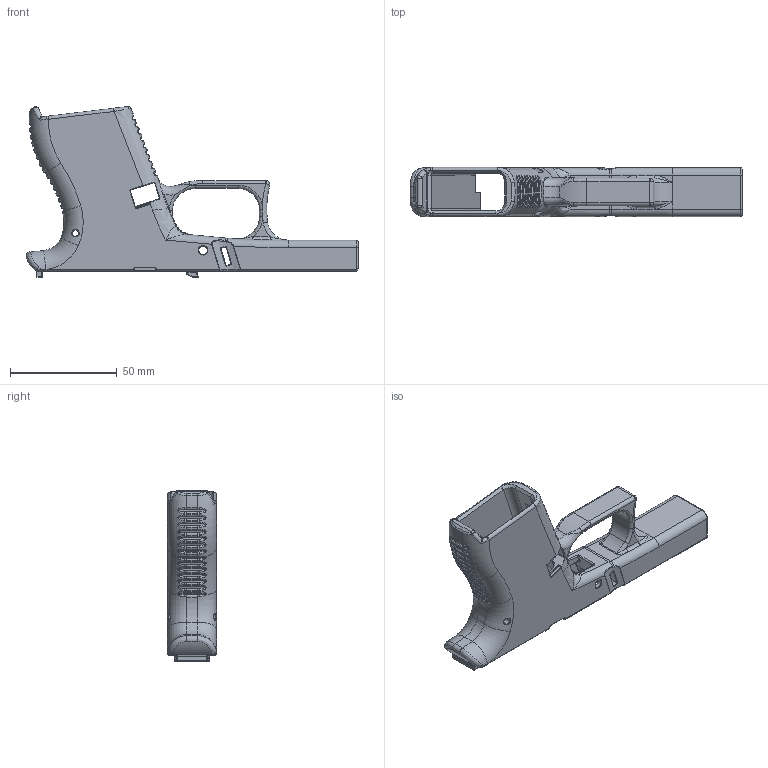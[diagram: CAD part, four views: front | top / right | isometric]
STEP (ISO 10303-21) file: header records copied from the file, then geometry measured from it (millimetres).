
FILE_DESCRIPTION(/* description */ (''),/* implementation_level */ '2;1');
FILE_NAME(/* name */ '23eda23c-9b73-40d3-b3ed-fe795d71b097.stp',/* time_stamp */ '2019-05-26T20:03:47-04:00',/* author */ ('suzuki450ltr'),/* organization */ (''),/* preprocessor_version */ 'ST-DEVELOPER v18',/* originating_system */ 'Autodesk Translation Framework v8.2.0.1029',/* authorisation */ '');
FILE_SCHEMA (('AUTOMOTIVE_DESIGN { 1 0 10303 214 3 1 1 }'));
Products named in the file (1): Glock 43 SS80
Bounding box: 155.83 x 23 x 80.21 mm (x, y, z)
Volume: 50057.9 mm3; surface area: 31982.8 mm2
Topology: 1 solids, 1 shells, 1341 faces, 3197 edges, 1786 vertices
Faces by surface type: bspline 545, cylinder 422, plane 201, torus 122, sphere 29, cone 22
Full cylindrical faces by diameter (mm): 3 x2, 3.5 x1, 4 x2
Entity records: 52659 total; most frequent: CARTESIAN_POINT 24643, ORIENTED_EDGE 6274, DIRECTION 5212, EDGE_CURVE 3137, AXIS2_PLACEMENT_3D 2124, VERTEX_POINT 1786, EDGE_LOOP 1351, FACE_OUTER_BOUND 1341
